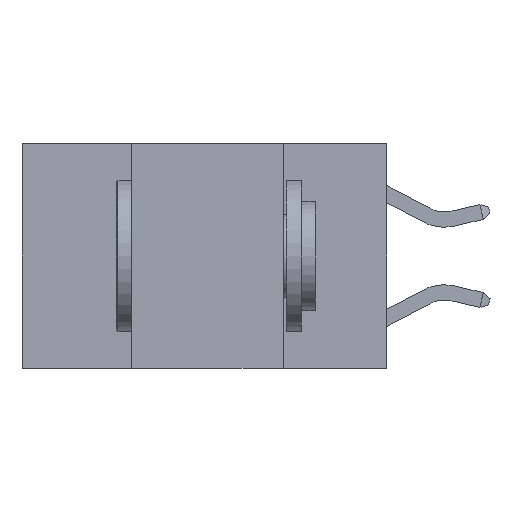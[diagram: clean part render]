
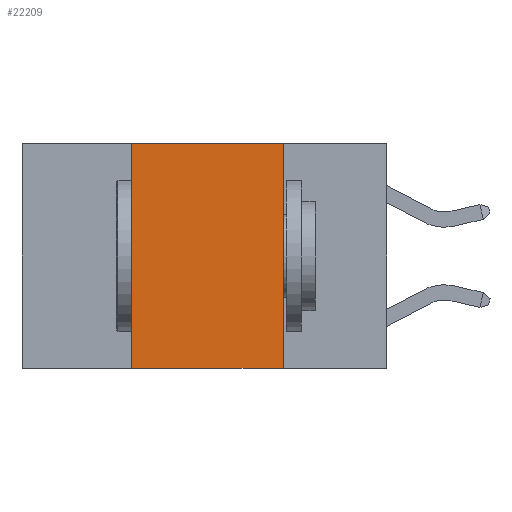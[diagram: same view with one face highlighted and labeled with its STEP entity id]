
A CAD part, left-side view. The second image highlights one B-rep face of the part: STEP entity #22209.
In plain terms, the highlighted planar face has unit normal (-1, 0, 0).
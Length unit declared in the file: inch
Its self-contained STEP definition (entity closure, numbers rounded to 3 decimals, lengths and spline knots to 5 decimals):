
#28 = LINE ( 'NONE', #1686, #13405 ) ;
#848 = VERTEX_POINT ( 'NONE', #20147 ) ;
#1268 = DIRECTION ( 'NONE',  ( 0., 0., -1. ) ) ;
#1686 = CARTESIAN_POINT ( 'NONE',  ( 0., 0.6, -0.37 ) ) ;
#4163 = VERTEX_POINT ( 'NONE', #19124 ) ;
#6724 = PLANE ( 'NONE',  #31911 ) ;
#7563 = CARTESIAN_POINT ( 'NONE',  ( 0., 0.17, 0. ) ) ;
#7606 = EDGE_CURVE ( 'NONE', #848, #4163, #29041, .T. ) ;
#7843 = CARTESIAN_POINT ( 'NONE',  ( 0., 0.17, -0.37 ) ) ;
#9399 = VECTOR ( 'NONE', #19327, 39.37008 ) ;
#10365 = ORIENTED_EDGE ( 'NONE', *, *, #25822, .F. ) ;
#10888 = LINE ( 'NONE', #30934, #23240 ) ;
#11755 = DIRECTION ( 'NONE',  ( 0., 0., -1. ) ) ;
#11802 = VECTOR ( 'NONE', #25614, 39.37008 ) ;
#13405 = VECTOR ( 'NONE', #19129, 39.37008 ) ;
#13514 = ORIENTED_EDGE ( 'NONE', *, *, #17576, .T. ) ;
#13901 = FACE_OUTER_BOUND ( 'NONE', #22381, .T. ) ;
#14000 = VERTEX_POINT ( 'NONE', #7843 ) ;
#16829 = CARTESIAN_POINT ( 'NONE',  ( 0., 0.42, 0. ) ) ;
#17576 = EDGE_CURVE ( 'NONE', #848, #14000, #28, .T. ) ;
#18320 = CARTESIAN_POINT ( 'NONE',  ( 0., 0.6, 0. ) ) ;
#18811 = EDGE_CURVE ( 'NONE', #4163, #21814, #31409, .T. ) ;
#19124 = CARTESIAN_POINT ( 'NONE',  ( 0., 0.42, 0. ) ) ;
#19129 = DIRECTION ( 'NONE',  ( 0., -1., 0. ) ) ;
#19283 = ORIENTED_EDGE ( 'NONE', *, *, #7606, .F. ) ;
#19327 = DIRECTION ( 'NONE',  ( 0., 0., 1. ) ) ;
#20147 = CARTESIAN_POINT ( 'NONE',  ( 0., 0.42, -0.37 ) ) ;
#21814 = VERTEX_POINT ( 'NONE', #7563 ) ;
#22209 = ADVANCED_FACE ( 'NONE', ( #13901 ), #6724, .F. ) ;
#22381 = EDGE_LOOP ( 'NONE', ( #10365, #31544, #19283, #13514 ) ) ;
#23240 = VECTOR ( 'NONE', #1268, 39.37008 ) ;
#25614 = DIRECTION ( 'NONE',  ( 0., -1., 0. ) ) ;
#25822 = EDGE_CURVE ( 'NONE', #21814, #14000, #10888, .T. ) ;
#26506 = DIRECTION ( 'NONE',  ( 1., 0., 0. ) ) ;
#28753 = CARTESIAN_POINT ( 'NONE',  ( 0., 0.6, 0. ) ) ;
#29041 = LINE ( 'NONE', #16829, #9399 ) ;
#30934 = CARTESIAN_POINT ( 'NONE',  ( 0., 0.17, 0. ) ) ;
#31409 = LINE ( 'NONE', #18320, #11802 ) ;
#31544 = ORIENTED_EDGE ( 'NONE', *, *, #18811, .F. ) ;
#31911 = AXIS2_PLACEMENT_3D ( 'NONE', #28753, #26506, #11755 ) ;
